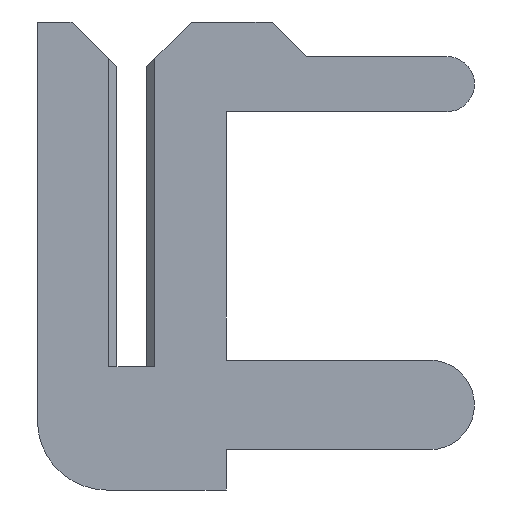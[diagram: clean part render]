
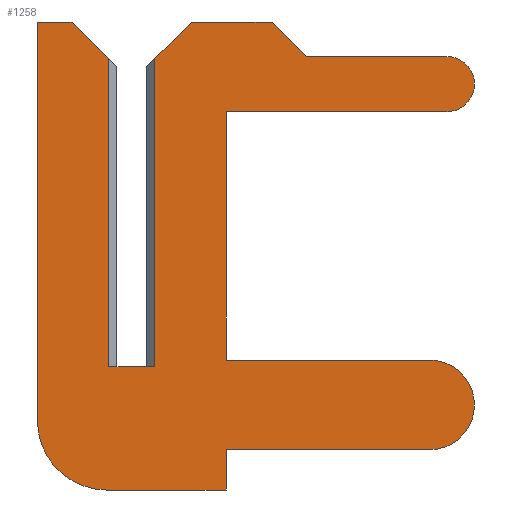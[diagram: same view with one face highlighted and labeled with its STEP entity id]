
A CAD part, left-side view. The second image highlights one B-rep face of the part: STEP entity #1258.
In plain terms, the highlighted planar face has unit normal (-1, 0, 0).
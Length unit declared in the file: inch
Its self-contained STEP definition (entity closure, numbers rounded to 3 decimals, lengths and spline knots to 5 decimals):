
#1 = CARTESIAN_POINT ( 'NONE',  ( -0.01, -0.0065, 0.1305 ) ) ;
#2 = DIRECTION ( 'NONE',  ( 0., 1., 0. ) ) ;
#17 = VECTOR ( 'NONE', #543, 39.37008 ) ;
#19 = LINE ( 'NONE', #1033, #309 ) ;
#22 = LINE ( 'NONE', #821, #496 ) ;
#33 = DIRECTION ( 'NONE',  ( 0., -1., 0. ) ) ;
#38 = EDGE_CURVE ( 'NONE', #637, #254, #1607, .T. ) ;
#39 = CARTESIAN_POINT ( 'NONE',  ( -0.01, -0.01, 0.134 ) ) ;
#46 = VERTEX_POINT ( 'NONE', #1246 ) ;
#62 = DIRECTION ( 'NONE',  ( 0., -1., 0. ) ) ;
#75 = VERTEX_POINT ( 'NONE', #268 ) ;
#85 = EDGE_CURVE ( 'NONE', #87, #358, #22, .T. ) ;
#87 = VERTEX_POINT ( 'NONE', #1131 ) ;
#121 = CARTESIAN_POINT ( 'NONE',  ( -0.01, -0.041, 0.003 ) ) ;
#124 = LINE ( 'NONE', #813, #1335 ) ;
#130 = EDGE_CURVE ( 'NONE', #530, #358, #412, .T. ) ;
#132 = DIRECTION ( 'NONE',  ( 0., 0., 1. ) ) ;
#135 = DIRECTION ( 'NONE',  ( 0., -0.707, -0.707 ) ) ;
#136 = ORIENTED_EDGE ( 'NONE', *, *, #1482, .T. ) ;
#144 = DIRECTION ( 'NONE',  ( 0., 0., 1. ) ) ;
#149 = LINE ( 'NONE', #875, #172 ) ;
#157 = ORIENTED_EDGE ( 'NONE', *, *, #521, .F. ) ;
#172 = VECTOR ( 'NONE', #1579, 39.37008 ) ;
#185 = EDGE_CURVE ( 'NONE', #1062, #928, #124, .T. ) ;
#196 = EDGE_CURVE ( 'NONE', #254, #1062, #1211, .T. ) ;
#201 = AXIS2_PLACEMENT_3D ( 'NONE', #717, #1150, #303 ) ;
#245 = EDGE_CURVE ( 'NONE', #928, #1346, #285, .T. ) ;
#254 = VERTEX_POINT ( 'NONE', #435 ) ;
#268 = CARTESIAN_POINT ( 'NONE',  ( -0.01, -0.061, 0.15 ) ) ;
#283 = CIRCLE ( 'NONE', #1276, 0.012 ) ;
#285 = CIRCLE ( 'NONE', #201, 0.03 ) ;
#292 = ORIENTED_EDGE ( 'NONE', *, *, #460, .F. ) ;
#293 = DIRECTION ( 'NONE',  ( 0., 0., 1. ) ) ;
#303 = DIRECTION ( 'NONE',  ( 0., 0., 1. ) ) ;
#307 = FACE_OUTER_BOUND ( 'NONE', #1320, .T. ) ;
#308 = DIRECTION ( 'NONE',  ( 0., 0., -1. ) ) ;
#309 = VECTOR ( 'NONE', #1727, 39.37008 ) ;
#311 = DIRECTION ( 'NONE',  ( 0., 0., -1. ) ) ;
#324 = CARTESIAN_POINT ( 'NONE',  ( -0.01, -0.026, 0.15 ) ) ;
#326 = VECTOR ( 'NONE', #308, 39.37008 ) ;
#344 = LINE ( 'NONE', #1430, #495 ) ;
#346 = LINE ( 'NONE', #324, #1522 ) ;
#358 = VERTEX_POINT ( 'NONE', #1707 ) ;
#366 = LINE ( 'NONE', #751, #1312 ) ;
#392 = CARTESIAN_POINT ( 'NONE',  ( -0.01, 0.026, 0.15 ) ) ;
#398 = CARTESIAN_POINT ( 'NONE',  ( -0.01, -0.1295, -0.0165 ) ) ;
#412 = LINE ( 'NONE', #1418, #1483 ) ;
#417 = EDGE_CURVE ( 'NONE', #833, #908, #669, .T. ) ;
#430 = ORIENTED_EDGE ( 'NONE', *, *, #1172, .F. ) ;
#435 = CARTESIAN_POINT ( 'NONE',  ( -0.01, -0.041, -0.036 ) ) ;
#443 = DIRECTION ( 'NONE',  ( 1., 0., 0. ) ) ;
#450 = ORIENTED_EDGE ( 'NONE', *, *, #130, .T. ) ;
#455 = VECTOR ( 'NONE', #311, 39.37008 ) ;
#460 = EDGE_CURVE ( 'NONE', #1346, #528, #19, .T. ) ;
#461 = VERTEX_POINT ( 'NONE', #39 ) ;
#485 = VERTEX_POINT ( 'NONE', #1013 ) ;
#495 = VECTOR ( 'NONE', #588, 39.37008 ) ;
#496 = VECTOR ( 'NONE', #135, 39.37008 ) ;
#510 = VERTEX_POINT ( 'NONE', #1444 ) ;
#521 = EDGE_CURVE ( 'NONE', #46, #75, #346, .T. ) ;
#528 = VERTEX_POINT ( 'NONE', #1022 ) ;
#530 = VERTEX_POINT ( 'NONE', #594 ) ;
#536 = LINE ( 'NONE', #1, #17 ) ;
#543 = DIRECTION ( 'NONE',  ( 0., -0.707, 0.707 ) ) ;
#559 = DIRECTION ( 'NONE',  ( 0., -0.707, -0.707 ) ) ;
#564 = CARTESIAN_POINT ( 'NONE',  ( -0.01, -0.041, 0.111 ) ) ;
#588 = DIRECTION ( 'NONE',  ( 0., -1., 0. ) ) ;
#593 = ORIENTED_EDGE ( 'NONE', *, *, #85, .F. ) ;
#594 = CARTESIAN_POINT ( 'NONE',  ( -0.01, 0.01, 0. ) ) ;
#617 = ORIENTED_EDGE ( 'NONE', *, *, #619, .F. ) ;
#619 = EDGE_CURVE ( 'NONE', #1251, #510, #344, .T. ) ;
#637 = VERTEX_POINT ( 'NONE', #1569 ) ;
#669 = LINE ( 'NONE', #886, #981 ) ;
#680 = EDGE_CURVE ( 'NONE', #530, #1496, #149, .T. ) ;
#717 = CARTESIAN_POINT ( 'NONE',  ( -0.01, 0.011, -0.0235 ) ) ;
#724 = ORIENTED_EDGE ( 'NONE', *, *, #185, .F. ) ;
#730 = DIRECTION ( 'NONE',  ( 0., 0., -1. ) ) ;
#751 = CARTESIAN_POINT ( 'NONE',  ( -0.01, -0.041, 0.003 ) ) ;
#759 = AXIS2_PLACEMENT_3D ( 'NONE', #1669, #820, #144 ) ;
#802 = EDGE_CURVE ( 'NONE', #528, #87, #846, .T. ) ;
#813 = CARTESIAN_POINT ( 'NONE',  ( -0.01, 0.011, -0.0535 ) ) ;
#820 = DIRECTION ( 'NONE',  ( -1., 0., 0. ) ) ;
#821 = CARTESIAN_POINT ( 'NONE',  ( -0.01, 0.0065, 0.1305 ) ) ;
#828 = CARTESIAN_POINT ( 'NONE',  ( -0.01, -0.041, -0.036 ) ) ;
#833 = VERTEX_POINT ( 'NONE', #1636 ) ;
#846 = LINE ( 'NONE', #392, #1291 ) ;
#869 = VECTOR ( 'NONE', #559, 39.37008 ) ;
#875 = CARTESIAN_POINT ( 'NONE',  ( -0.01, 0.0065, 0. ) ) ;
#886 = CARTESIAN_POINT ( 'NONE',  ( -0.01, -0.137, 0.135 ) ) ;
#908 = VERTEX_POINT ( 'NONE', #1502 ) ;
#928 = VERTEX_POINT ( 'NONE', #1361 ) ;
#941 = ORIENTED_EDGE ( 'NONE', *, *, #1446, .F. ) ;
#947 = ORIENTED_EDGE ( 'NONE', *, *, #417, .F. ) ;
#954 = CARTESIAN_POINT ( 'NONE',  ( -0.01, 0.041, -0.0235 ) ) ;
#981 = VECTOR ( 'NONE', #33, 39.37008 ) ;
#997 = ORIENTED_EDGE ( 'NONE', *, *, #680, .F. ) ;
#1013 = CARTESIAN_POINT ( 'NONE',  ( -0.01, -0.137, 0.111 ) ) ;
#1022 = CARTESIAN_POINT ( 'NONE',  ( -0.01, 0.041, 0.15 ) ) ;
#1033 = CARTESIAN_POINT ( 'NONE',  ( -0.01, 0.041, 0.15 ) ) ;
#1037 = VERTEX_POINT ( 'NONE', #1239 ) ;
#1062 = VERTEX_POINT ( 'NONE', #1195 ) ;
#1080 = EDGE_CURVE ( 'NONE', #510, #637, #1549, .T. ) ;
#1107 = ORIENTED_EDGE ( 'NONE', *, *, #1689, .F. ) ;
#1124 = DIRECTION ( 'NONE',  ( 0., 1., 0. ) ) ;
#1131 = CARTESIAN_POINT ( 'NONE',  ( -0.01, 0.026, 0.15 ) ) ;
#1150 = DIRECTION ( 'NONE',  ( 1., 0., 0. ) ) ;
#1172 = EDGE_CURVE ( 'NONE', #461, #46, #536, .T. ) ;
#1195 = CARTESIAN_POINT ( 'NONE',  ( -0.01, -0.041, -0.0535 ) ) ;
#1211 = LINE ( 'NONE', #1628, #455 ) ;
#1214 = EDGE_CURVE ( 'NONE', #75, #833, #1755, .T. ) ;
#1225 = ORIENTED_EDGE ( 'NONE', *, *, #1080, .F. ) ;
#1239 = CARTESIAN_POINT ( 'NONE',  ( -0.01, -0.041, 0.111 ) ) ;
#1246 = CARTESIAN_POINT ( 'NONE',  ( -0.01, -0.026, 0.15 ) ) ;
#1251 = VERTEX_POINT ( 'NONE', #121 ) ;
#1258 = ADVANCED_FACE ( 'NONE', ( #307 ), #1534, .T. ) ;
#1276 = AXIS2_PLACEMENT_3D ( 'NONE', #1429, #443, #293 ) ;
#1277 = CARTESIAN_POINT ( 'NONE',  ( -0.01, -0.01, 0.15 ) ) ;
#1286 = ORIENTED_EDGE ( 'NONE', *, *, #245, .F. ) ;
#1291 = VECTOR ( 'NONE', #62, 39.37008 ) ;
#1293 = DIRECTION ( 'NONE',  ( 0., 0., 1. ) ) ;
#1307 = AXIS2_PLACEMENT_3D ( 'NONE', #398, #1396, #132 ) ;
#1312 = VECTOR ( 'NONE', #730, 39.37008 ) ;
#1320 = EDGE_LOOP ( 'NONE', ( #430, #136, #997, #450, #593, #1765, #292, #1286, #724, #1382, #1509, #1225, #617, #1107, #1584, #941, #947, #1624, #157 ) ) ;
#1330 = LINE ( 'NONE', #1277, #326 ) ;
#1335 = VECTOR ( 'NONE', #2, 39.37008 ) ;
#1346 = VERTEX_POINT ( 'NONE', #954 ) ;
#1361 = CARTESIAN_POINT ( 'NONE',  ( -0.01, 0.011, -0.0535 ) ) ;
#1382 = ORIENTED_EDGE ( 'NONE', *, *, #196, .F. ) ;
#1396 = DIRECTION ( 'NONE',  ( 1., 0., 0. ) ) ;
#1418 = CARTESIAN_POINT ( 'NONE',  ( -0.01, 0.01, -0.0235 ) ) ;
#1429 = CARTESIAN_POINT ( 'NONE',  ( -0.01, -0.137, 0.123 ) ) ;
#1430 = CARTESIAN_POINT ( 'NONE',  ( -0.01, -0.1295, 0.003 ) ) ;
#1444 = CARTESIAN_POINT ( 'NONE',  ( -0.01, -0.1295, 0.003 ) ) ;
#1446 = EDGE_CURVE ( 'NONE', #908, #485, #283, .T. ) ;
#1482 = EDGE_CURVE ( 'NONE', #461, #1496, #1330, .T. ) ;
#1483 = VECTOR ( 'NONE', #1293, 39.37008 ) ;
#1496 = VERTEX_POINT ( 'NONE', #1550 ) ;
#1502 = CARTESIAN_POINT ( 'NONE',  ( -0.01, -0.137, 0.135 ) ) ;
#1509 = ORIENTED_EDGE ( 'NONE', *, *, #38, .F. ) ;
#1522 = VECTOR ( 'NONE', #1597, 39.37008 ) ;
#1526 = CARTESIAN_POINT ( 'NONE',  ( -0.01, -0.076, 0.135 ) ) ;
#1534 = PLANE ( 'NONE',  #759 ) ;
#1549 = CIRCLE ( 'NONE', #1307, 0.0195 ) ;
#1550 = CARTESIAN_POINT ( 'NONE',  ( -0.01, -0.01, 0. ) ) ;
#1562 = DIRECTION ( 'NONE',  ( 0., 1., 0. ) ) ;
#1569 = CARTESIAN_POINT ( 'NONE',  ( -0.01, -0.1295, -0.036 ) ) ;
#1576 = EDGE_CURVE ( 'NONE', #485, #1037, #1751, .T. ) ;
#1579 = DIRECTION ( 'NONE',  ( 0., -1., 0. ) ) ;
#1584 = ORIENTED_EDGE ( 'NONE', *, *, #1576, .F. ) ;
#1597 = DIRECTION ( 'NONE',  ( 0., -1., 0. ) ) ;
#1607 = LINE ( 'NONE', #828, #1729 ) ;
#1624 = ORIENTED_EDGE ( 'NONE', *, *, #1214, .F. ) ;
#1628 = CARTESIAN_POINT ( 'NONE',  ( -0.01, -0.041, -0.0535 ) ) ;
#1636 = CARTESIAN_POINT ( 'NONE',  ( -0.01, -0.076, 0.135 ) ) ;
#1657 = VECTOR ( 'NONE', #1562, 39.37008 ) ;
#1669 = CARTESIAN_POINT ( 'NONE',  ( -0.01, 0.011, -0.0235 ) ) ;
#1689 = EDGE_CURVE ( 'NONE', #1037, #1251, #366, .T. ) ;
#1707 = CARTESIAN_POINT ( 'NONE',  ( -0.01, 0.01, 0.134 ) ) ;
#1727 = DIRECTION ( 'NONE',  ( 0., 0., 1. ) ) ;
#1729 = VECTOR ( 'NONE', #1124, 39.37008 ) ;
#1751 = LINE ( 'NONE', #564, #1657 ) ;
#1755 = LINE ( 'NONE', #1526, #869 ) ;
#1765 = ORIENTED_EDGE ( 'NONE', *, *, #802, .F. ) ;
